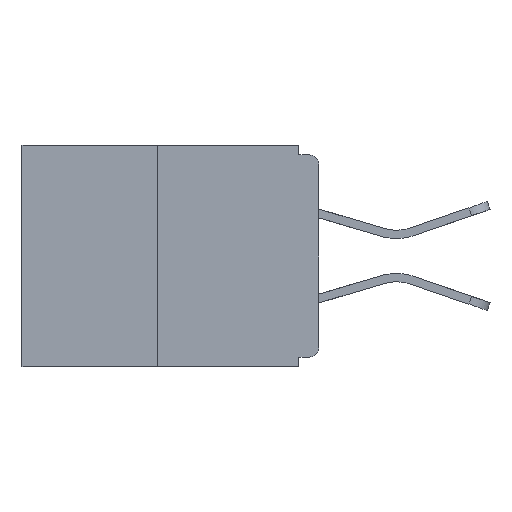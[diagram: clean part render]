
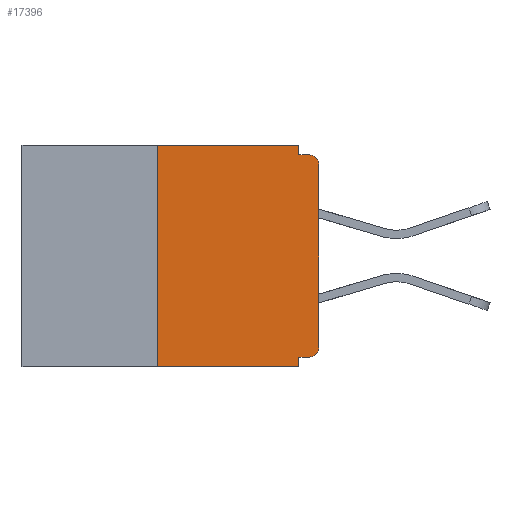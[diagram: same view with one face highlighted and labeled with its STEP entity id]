
A CAD part, left-side view. The second image highlights one B-rep face of the part: STEP entity #17396.
In plain terms, the highlighted planar face has unit normal (-1, 0, 0).
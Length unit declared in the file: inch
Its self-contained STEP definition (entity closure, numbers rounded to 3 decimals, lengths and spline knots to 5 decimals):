
#227 = VECTOR ( 'NONE', #4637, 39.37008 ) ;
#297 = CARTESIAN_POINT ( 'NONE',  ( 0., 0., -0.03 ) ) ;
#397 = ORIENTED_EDGE ( 'NONE', *, *, #4249, .T. ) ;
#410 = CARTESIAN_POINT ( 'NONE',  ( 0., 0.031, -0.343 ) ) ;
#484 = CARTESIAN_POINT ( 'NONE',  ( 0., 0.031, 0. ) ) ;
#944 = ORIENTED_EDGE ( 'NONE', *, *, #9448, .F. ) ;
#1670 = VERTEX_POINT ( 'NONE', #11311 ) ;
#2298 = EDGE_CURVE ( 'NONE', #13498, #6672, #21665, .T. ) ;
#3053 = DIRECTION ( 'NONE',  ( 0., 0., -1. ) ) ;
#3194 = ORIENTED_EDGE ( 'NONE', *, *, #17161, .F. ) ;
#3541 = ORIENTED_EDGE ( 'NONE', *, *, #9572, .F. ) ;
#3905 = VERTEX_POINT ( 'NONE', #13439 ) ;
#4028 = VECTOR ( 'NONE', #7616, 39.37008 ) ;
#4249 = EDGE_CURVE ( 'NONE', #1670, #3905, #11696, .T. ) ;
#4553 = DIRECTION ( 'NONE',  ( -1., 0., 0. ) ) ;
#4580 = LINE ( 'NONE', #18504, #4028 ) ;
#4637 = DIRECTION ( 'NONE',  ( 0., -1., 0. ) ) ;
#4721 = CARTESIAN_POINT ( 'NONE',  ( 0., 0.031, -0.015 ) ) ;
#5007 = ORIENTED_EDGE ( 'NONE', *, *, #21872, .T. ) ;
#5044 = VECTOR ( 'NONE', #8210, 39.37008 ) ;
#5232 = LINE ( 'NONE', #8475, #19390 ) ;
#5253 = EDGE_LOOP ( 'NONE', ( #22677, #944, #23218, #3194, #3541, #397, #5007, #16077, #23704, #17165 ) ) ;
#5719 = VERTEX_POINT ( 'NONE', #410 ) ;
#5846 = AXIS2_PLACEMENT_3D ( 'NONE', #22506, #17598, #23736 ) ;
#5892 = VECTOR ( 'NONE', #16324, 39.37008 ) ;
#6075 = VERTEX_POINT ( 'NONE', #14466 ) ;
#6243 = EDGE_CURVE ( 'NONE', #8868, #6075, #8436, .T. ) ;
#6672 = VERTEX_POINT ( 'NONE', #7251 ) ;
#7171 = VECTOR ( 'NONE', #18576, 39.37008 ) ;
#7251 = CARTESIAN_POINT ( 'NONE',  ( 0., 0.031, 0. ) ) ;
#7616 = DIRECTION ( 'NONE',  ( 0., 0., 1. ) ) ;
#8037 = CARTESIAN_POINT ( 'NONE',  ( 0., 0.031, -0.328 ) ) ;
#8210 = DIRECTION ( 'NONE',  ( 0., 0., -1. ) ) ;
#8436 = LINE ( 'NONE', #17462, #21439 ) ;
#8470 = LINE ( 'NONE', #10662, #5892 ) ;
#8475 = CARTESIAN_POINT ( 'NONE',  ( 0., 0.031, -0.343 ) ) ;
#8868 = VERTEX_POINT ( 'NONE', #4721 ) ;
#9448 = EDGE_CURVE ( 'NONE', #16249, #13498, #16995, .T. ) ;
#9572 = EDGE_CURVE ( 'NONE', #1670, #15543, #19301, .T. ) ;
#10242 = CARTESIAN_POINT ( 'NONE',  ( 0., 0.46, 0. ) ) ;
#10474 = PLANE ( 'NONE',  #15777 ) ;
#10662 = CARTESIAN_POINT ( 'NONE',  ( 0., 0.46, -0.343 ) ) ;
#11310 = CARTESIAN_POINT ( 'NONE',  ( 0., 0.015, -0.03 ) ) ;
#11311 = CARTESIAN_POINT ( 'NONE',  ( 0., 0.015, -0.328 ) ) ;
#11685 = CARTESIAN_POINT ( 'NONE',  ( 0., 0.25, 0. ) ) ;
#11696 = CIRCLE ( 'NONE', #5846, 0.015 ) ;
#13112 = AXIS2_PLACEMENT_3D ( 'NONE', #11310, #4553, #23025 ) ;
#13439 = CARTESIAN_POINT ( 'NONE',  ( 0., 0., -0.313 ) ) ;
#13498 = VERTEX_POINT ( 'NONE', #11685 ) ;
#13672 = CARTESIAN_POINT ( 'NONE',  ( 0., 0.46, 0. ) ) ;
#13875 = FACE_OUTER_BOUND ( 'NONE', #5253, .T. ) ;
#14111 = DIRECTION ( 'NONE',  ( 0., 0., -1. ) ) ;
#14215 = DIRECTION ( 'NONE',  ( 1., 0., 0. ) ) ;
#14390 = VECTOR ( 'NONE', #21087, 39.37008 ) ;
#14466 = CARTESIAN_POINT ( 'NONE',  ( 0., 0.015, -0.015 ) ) ;
#14480 = EDGE_CURVE ( 'NONE', #6672, #8868, #15167, .T. ) ;
#14783 = CARTESIAN_POINT ( 'NONE',  ( 0., 0.25, 0. ) ) ;
#15167 = LINE ( 'NONE', #484, #5044 ) ;
#15543 = VERTEX_POINT ( 'NONE', #8037 ) ;
#15777 = AXIS2_PLACEMENT_3D ( 'NONE', #10242, #14215, #3053 ) ;
#16077 = ORIENTED_EDGE ( 'NONE', *, *, #18019, .T. ) ;
#16249 = VERTEX_POINT ( 'NONE', #19037 ) ;
#16324 = DIRECTION ( 'NONE',  ( 0., -1., 0. ) ) ;
#16995 = LINE ( 'NONE', #14783, #7171 ) ;
#17161 = EDGE_CURVE ( 'NONE', #15543, #5719, #5232, .T. ) ;
#17165 = ORIENTED_EDGE ( 'NONE', *, *, #14480, .F. ) ;
#17396 = ADVANCED_FACE ( 'NONE', ( #13875 ), #10474, .F. ) ;
#17462 = CARTESIAN_POINT ( 'NONE',  ( 0., 0., -0.015 ) ) ;
#17598 = DIRECTION ( 'NONE',  ( -1., 0., 0. ) ) ;
#18019 = EDGE_CURVE ( 'NONE', #19533, #6075, #20658, .T. ) ;
#18504 = CARTESIAN_POINT ( 'NONE',  ( 0., 0., 0. ) ) ;
#18576 = DIRECTION ( 'NONE',  ( 0., 0., 1. ) ) ;
#19037 = CARTESIAN_POINT ( 'NONE',  ( 0., 0.25, -0.343 ) ) ;
#19219 = EDGE_CURVE ( 'NONE', #16249, #5719, #8470, .T. ) ;
#19301 = LINE ( 'NONE', #19380, #14390 ) ;
#19380 = CARTESIAN_POINT ( 'NONE',  ( 0., 0., -0.328 ) ) ;
#19390 = VECTOR ( 'NONE', #14111, 39.37008 ) ;
#19533 = VERTEX_POINT ( 'NONE', #297 ) ;
#20658 = CIRCLE ( 'NONE', #13112, 0.015 ) ;
#21087 = DIRECTION ( 'NONE',  ( 0., 1., 0. ) ) ;
#21439 = VECTOR ( 'NONE', #23122, 39.37008 ) ;
#21665 = LINE ( 'NONE', #13672, #227 ) ;
#21872 = EDGE_CURVE ( 'NONE', #3905, #19533, #4580, .T. ) ;
#22506 = CARTESIAN_POINT ( 'NONE',  ( 0., 0.015, -0.313 ) ) ;
#22677 = ORIENTED_EDGE ( 'NONE', *, *, #2298, .F. ) ;
#23025 = DIRECTION ( 'NONE',  ( 0., 0., -1. ) ) ;
#23122 = DIRECTION ( 'NONE',  ( 0., -1., 0. ) ) ;
#23218 = ORIENTED_EDGE ( 'NONE', *, *, #19219, .T. ) ;
#23704 = ORIENTED_EDGE ( 'NONE', *, *, #6243, .F. ) ;
#23736 = DIRECTION ( 'NONE',  ( 0., 0., -1. ) ) ;
